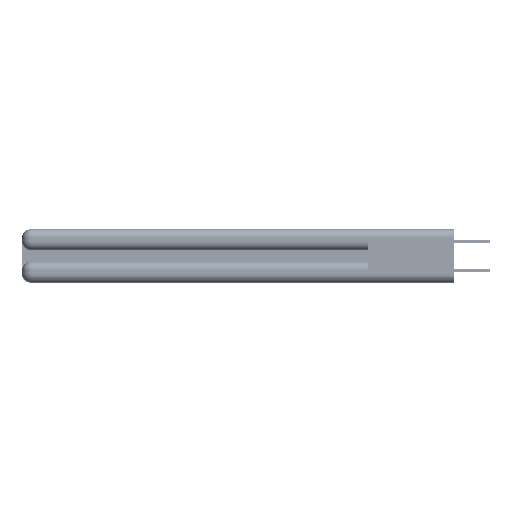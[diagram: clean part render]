
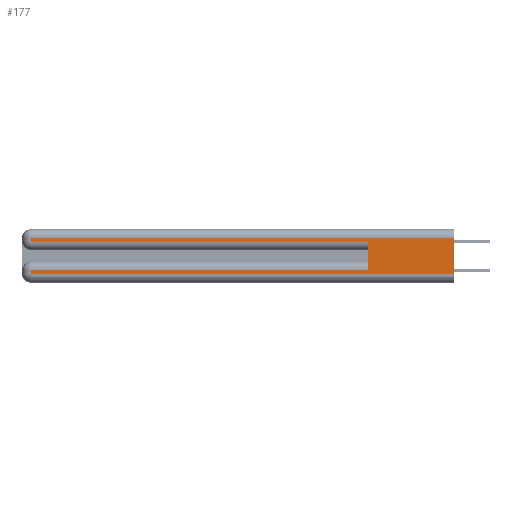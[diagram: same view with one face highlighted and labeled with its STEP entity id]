
A CAD part, left-side view. The second image highlights one B-rep face of the part: STEP entity #177.
In plain terms, the highlighted planar face has unit normal (-1, 0, 0).
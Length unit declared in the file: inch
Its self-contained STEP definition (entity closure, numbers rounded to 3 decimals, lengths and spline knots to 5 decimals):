
#177 = ADVANCED_FACE ( 'NONE', ( #15405 ), #6437, .F. ) ;
#749 = CARTESIAN_POINT ( 'NONE',  ( 0., 0., 0.37 ) ) ;
#1782 = CARTESIAN_POINT ( 'NONE',  ( 0., 2.94, 0.06 ) ) ;
#3153 = DIRECTION ( 'NONE',  ( 0., 0., -1. ) ) ;
#4712 = ORIENTED_EDGE ( 'NONE', *, *, #14891, .F. ) ;
#4807 = VECTOR ( 'NONE', #10241, 39.37008 ) ;
#6437 = PLANE ( 'NONE',  #26689 ) ;
#6461 = VERTEX_POINT ( 'NONE', #42778 ) ;
#7073 = ORIENTED_EDGE ( 'NONE', *, *, #39721, .T. ) ;
#7676 = DIRECTION ( 'NONE',  ( 0., -1., 0. ) ) ;
#9382 = CARTESIAN_POINT ( 'NONE',  ( 0., 0., 0.31 ) ) ;
#9480 = DIRECTION ( 'NONE',  ( 1., 0., 0. ) ) ;
#9830 = VERTEX_POINT ( 'NONE', #9382 ) ;
#10241 = DIRECTION ( 'NONE',  ( 0., 0., -1. ) ) ;
#10873 = LINE ( 'NONE', #18796, #36826 ) ;
#11162 = CARTESIAN_POINT ( 'NONE',  ( 0., 0.6, 0.085 ) ) ;
#11714 = VECTOR ( 'NONE', #23577, 39.37008 ) ;
#13044 = VECTOR ( 'NONE', #7676, 39.37008 ) ;
#13684 = CARTESIAN_POINT ( 'NONE',  ( 0., 2.94, 0.37 ) ) ;
#14400 = ORIENTED_EDGE ( 'NONE', *, *, #24607, .T. ) ;
#14891 = EDGE_CURVE ( 'NONE', #9830, #17089, #34261, .T. ) ;
#15405 = FACE_OUTER_BOUND ( 'NONE', #24203, .T. ) ;
#17089 = VERTEX_POINT ( 'NONE', #31509 ) ;
#18505 = ORIENTED_EDGE ( 'NONE', *, *, #41064, .T. ) ;
#18796 = CARTESIAN_POINT ( 'NONE',  ( 0., 2.94, 0.37 ) ) ;
#19175 = LINE ( 'NONE', #35933, #42348 ) ;
#20054 = LINE ( 'NONE', #25048, #13044 ) ;
#21803 = DIRECTION ( 'NONE',  ( 0., 0., 1. ) ) ;
#23577 = DIRECTION ( 'NONE',  ( 0., 1., 0. ) ) ;
#23645 = CARTESIAN_POINT ( 'NONE',  ( 0., 0., 0.37 ) ) ;
#24203 = EDGE_LOOP ( 'NONE', ( #4712, #18505, #7073, #30156, #33274, #40913, #31396, #14400 ) ) ;
#24514 = CARTESIAN_POINT ( 'NONE',  ( 0., 0., 0.06 ) ) ;
#24607 = EDGE_CURVE ( 'NONE', #29983, #17089, #43328, .T. ) ;
#25039 = VECTOR ( 'NONE', #28345, 39.37008 ) ;
#25048 = CARTESIAN_POINT ( 'NONE',  ( 0., 0., 0.285 ) ) ;
#25813 = DIRECTION ( 'NONE',  ( 0., 1., 0. ) ) ;
#26080 = VERTEX_POINT ( 'NONE', #34183 ) ;
#26689 = AXIS2_PLACEMENT_3D ( 'NONE', #23645, #9480, #3153 ) ;
#27709 = VERTEX_POINT ( 'NONE', #11162 ) ;
#27992 = DIRECTION ( 'NONE',  ( 0., -1., 0. ) ) ;
#28174 = VECTOR ( 'NONE', #27992, 39.37008 ) ;
#28318 = EDGE_CURVE ( 'NONE', #44497, #31146, #20054, .T. ) ;
#28345 = DIRECTION ( 'NONE',  ( 0., 0., -1. ) ) ;
#29071 = DIRECTION ( 'NONE',  ( 0., 0., -1. ) ) ;
#29983 = VERTEX_POINT ( 'NONE', #1782 ) ;
#30156 = ORIENTED_EDGE ( 'NONE', *, *, #28318, .T. ) ;
#30813 = CARTESIAN_POINT ( 'NONE',  ( 0., 0., 0.31 ) ) ;
#31109 = LINE ( 'NONE', #38874, #34887 ) ;
#31146 = VERTEX_POINT ( 'NONE', #38558 ) ;
#31283 = EDGE_CURVE ( 'NONE', #27709, #31146, #31109, .T. ) ;
#31396 = ORIENTED_EDGE ( 'NONE', *, *, #32521, .T. ) ;
#31509 = CARTESIAN_POINT ( 'NONE',  ( 0., 0., 0.06 ) ) ;
#32361 = CARTESIAN_POINT ( 'NONE',  ( 0., 2.94, 0.285 ) ) ;
#32521 = EDGE_CURVE ( 'NONE', #26080, #29983, #10873, .T. ) ;
#33274 = ORIENTED_EDGE ( 'NONE', *, *, #31283, .F. ) ;
#33963 = LINE ( 'NONE', #13684, #4807 ) ;
#34183 = CARTESIAN_POINT ( 'NONE',  ( 0., 2.94, 0.085 ) ) ;
#34261 = LINE ( 'NONE', #749, #25039 ) ;
#34887 = VECTOR ( 'NONE', #21803, 39.37008 ) ;
#35933 = CARTESIAN_POINT ( 'NONE',  ( 0., 0., 0.085 ) ) ;
#36826 = VECTOR ( 'NONE', #29071, 39.37008 ) ;
#38558 = CARTESIAN_POINT ( 'NONE',  ( 0., 0.6, 0.285 ) ) ;
#38874 = CARTESIAN_POINT ( 'NONE',  ( 0., 0.6, 0.145 ) ) ;
#39721 = EDGE_CURVE ( 'NONE', #6461, #44497, #33963, .T. ) ;
#40337 = LINE ( 'NONE', #30813, #11714 ) ;
#40913 = ORIENTED_EDGE ( 'NONE', *, *, #42627, .T. ) ;
#41064 = EDGE_CURVE ( 'NONE', #9830, #6461, #40337, .T. ) ;
#42348 = VECTOR ( 'NONE', #25813, 39.37008 ) ;
#42627 = EDGE_CURVE ( 'NONE', #27709, #26080, #19175, .T. ) ;
#42778 = CARTESIAN_POINT ( 'NONE',  ( 0., 2.94, 0.31 ) ) ;
#43328 = LINE ( 'NONE', #24514, #28174 ) ;
#44497 = VERTEX_POINT ( 'NONE', #32361 ) ;
